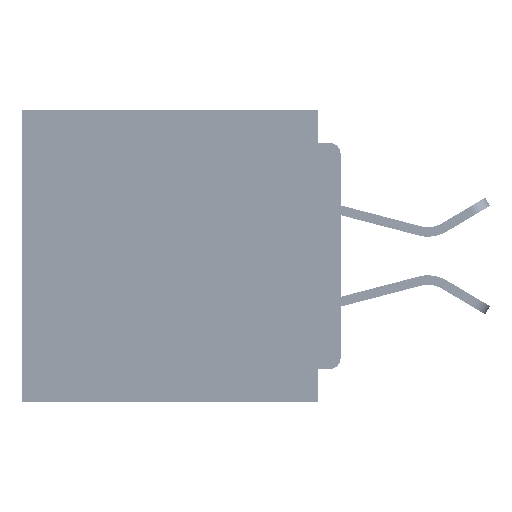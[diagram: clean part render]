
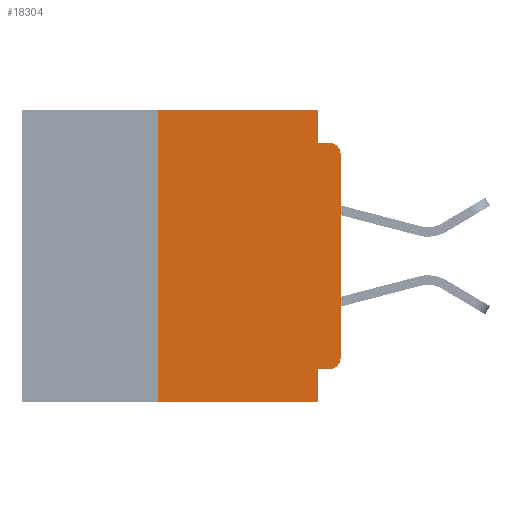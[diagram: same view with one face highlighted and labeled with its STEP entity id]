
A CAD part, left-side view. The second image highlights one B-rep face of the part: STEP entity #18304.
In plain terms, the highlighted planar face has unit normal (-1, 0, 0).
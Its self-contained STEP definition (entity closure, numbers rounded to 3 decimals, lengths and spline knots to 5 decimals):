
#236 = ORIENTED_EDGE ( 'NONE', *, *, #32184, .T. ) ;
#1156 = VERTEX_POINT ( 'NONE', #45394 ) ;
#2224 = ORIENTED_EDGE ( 'NONE', *, *, #14441, .F. ) ;
#2262 = LINE ( 'NONE', #34081, #57100 ) ;
#6101 = VERTEX_POINT ( 'NONE', #47348 ) ;
#6342 = ORIENTED_EDGE ( 'NONE', *, *, #63962, .F. ) ;
#6578 = DIRECTION ( 'NONE',  ( 0., 0., -1. ) ) ;
#8462 = VERTEX_POINT ( 'NONE', #50744 ) ;
#9074 = DIRECTION ( 'NONE',  ( 0., 0., -1. ) ) ;
#9329 = VERTEX_POINT ( 'NONE', #69823 ) ;
#13251 = LINE ( 'NONE', #45003, #56985 ) ;
#14441 = EDGE_CURVE ( 'NONE', #62537, #6101, #2262, .T. ) ;
#14449 = ORIENTED_EDGE ( 'NONE', *, *, #30788, .F. ) ;
#14772 = CARTESIAN_POINT ( 'NONE',  ( 0., 0.031, -0.4 ) ) ;
#15484 = VERTEX_POINT ( 'NONE', #60192 ) ;
#16236 = EDGE_CURVE ( 'NONE', #1156, #57946, #32919, .T. ) ;
#17476 = DIRECTION ( 'NONE',  ( 0., -1., 0. ) ) ;
#17561 = VECTOR ( 'NONE', #68040, 39.37008 ) ;
#18009 = DIRECTION ( 'NONE',  ( -1., 0., 0. ) ) ;
#18274 = VECTOR ( 'NONE', #17476, 39.37008 ) ;
#18304 = ADVANCED_FACE ( 'NONE', ( #35340 ), #30958, .F. ) ;
#18717 = CARTESIAN_POINT ( 'NONE',  ( 0., 0., -0.06 ) ) ;
#18816 = VECTOR ( 'NONE', #20303, 39.37008 ) ;
#18832 = CARTESIAN_POINT ( 'NONE',  ( 0., 0., -0.355 ) ) ;
#20011 = VECTOR ( 'NONE', #60569, 39.37008 ) ;
#20154 = CIRCLE ( 'NONE', #34259, 0.015 ) ;
#20303 = DIRECTION ( 'NONE',  ( 0., 0., -1. ) ) ;
#21872 = LINE ( 'NONE', #59383, #62013 ) ;
#22341 = CARTESIAN_POINT ( 'NONE',  ( 0., 0.25, -0.4 ) ) ;
#22811 = DIRECTION ( 'NONE',  ( 0., 0., 1. ) ) ;
#25427 = CARTESIAN_POINT ( 'NONE',  ( 0., 0.437, 0. ) ) ;
#26601 = CARTESIAN_POINT ( 'NONE',  ( 0., 0.25, 0. ) ) ;
#28005 = AXIS2_PLACEMENT_3D ( 'NONE', #50882, #18009, #56341 ) ;
#28533 = DIRECTION ( 'NONE',  ( 0., -1., 0. ) ) ;
#29160 = ORIENTED_EDGE ( 'NONE', *, *, #61108, .F. ) ;
#29450 = ORIENTED_EDGE ( 'NONE', *, *, #44768, .T. ) ;
#29690 = CARTESIAN_POINT ( 'NONE',  ( 0., 0., -0.34 ) ) ;
#30630 = DIRECTION ( 'NONE',  ( -1., 0., 0. ) ) ;
#30788 = EDGE_CURVE ( 'NONE', #6101, #8462, #13251, .T. ) ;
#30958 = PLANE ( 'NONE',  #44777 ) ;
#32147 = DIRECTION ( 'NONE',  ( 0., -1., 0. ) ) ;
#32184 = EDGE_CURVE ( 'NONE', #70499, #42153, #56794, .T. ) ;
#32205 = LINE ( 'NONE', #18832, #17561 ) ;
#32885 = LINE ( 'NONE', #22341, #20011 ) ;
#32919 = LINE ( 'NONE', #50360, #18274 ) ;
#34081 = CARTESIAN_POINT ( 'NONE',  ( 0., 0.437, 0. ) ) ;
#34259 = AXIS2_PLACEMENT_3D ( 'NONE', #63284, #30630, #68730 ) ;
#35340 = FACE_OUTER_BOUND ( 'NONE', #52729, .T. ) ;
#38305 = CARTESIAN_POINT ( 'NONE',  ( 0., 0.031, -0.4 ) ) ;
#40132 = EDGE_CURVE ( 'NONE', #9329, #70499, #68494, .T. ) ;
#40573 = VECTOR ( 'NONE', #22811, 39.37008 ) ;
#42026 = DIRECTION ( 'NONE',  ( 1., 0., 0. ) ) ;
#42153 = VERTEX_POINT ( 'NONE', #18717 ) ;
#44768 = EDGE_CURVE ( 'NONE', #42153, #63055, #20154, .T. ) ;
#44777 = AXIS2_PLACEMENT_3D ( 'NONE', #25427, #42026, #9074 ) ;
#45003 = CARTESIAN_POINT ( 'NONE',  ( 0., 0.031, 0. ) ) ;
#45394 = CARTESIAN_POINT ( 'NONE',  ( 0., 0.25, -0.4 ) ) ;
#45664 = EDGE_CURVE ( 'NONE', #1156, #62537, #32885, .T. ) ;
#46444 = ORIENTED_EDGE ( 'NONE', *, *, #66779, .F. ) ;
#47348 = CARTESIAN_POINT ( 'NONE',  ( 0., 0.031, 0. ) ) ;
#49178 = ORIENTED_EDGE ( 'NONE', *, *, #16236, .T. ) ;
#50360 = CARTESIAN_POINT ( 'NONE',  ( 0., 0.437, -0.4 ) ) ;
#50744 = CARTESIAN_POINT ( 'NONE',  ( 0., 0.031, -0.045 ) ) ;
#50882 = CARTESIAN_POINT ( 'NONE',  ( 0., 0.015, -0.34 ) ) ;
#52729 = EDGE_LOOP ( 'NONE', ( #236, #29450, #6342, #14449, #2224, #66175, #49178, #46444, #29160, #55626 ) ) ;
#55626 = ORIENTED_EDGE ( 'NONE', *, *, #40132, .T. ) ;
#56341 = DIRECTION ( 'NONE',  ( 0., 0., -1. ) ) ;
#56794 = LINE ( 'NONE', #61023, #40573 ) ;
#56985 = VECTOR ( 'NONE', #6578, 39.37008 ) ;
#57100 = VECTOR ( 'NONE', #28533, 39.37008 ) ;
#57946 = VERTEX_POINT ( 'NONE', #38305 ) ;
#58095 = CARTESIAN_POINT ( 'NONE',  ( 0., 0.015, -0.045 ) ) ;
#59383 = CARTESIAN_POINT ( 'NONE',  ( 0., 0., -0.045 ) ) ;
#60192 = CARTESIAN_POINT ( 'NONE',  ( 0., 0.031, -0.355 ) ) ;
#60569 = DIRECTION ( 'NONE',  ( 0., 0., 1. ) ) ;
#61023 = CARTESIAN_POINT ( 'NONE',  ( 0., 0., 0. ) ) ;
#61108 = EDGE_CURVE ( 'NONE', #9329, #15484, #32205, .T. ) ;
#62013 = VECTOR ( 'NONE', #32147, 39.37008 ) ;
#62427 = LINE ( 'NONE', #14772, #18816 ) ;
#62537 = VERTEX_POINT ( 'NONE', #26601 ) ;
#63055 = VERTEX_POINT ( 'NONE', #58095 ) ;
#63284 = CARTESIAN_POINT ( 'NONE',  ( 0., 0.015, -0.06 ) ) ;
#63962 = EDGE_CURVE ( 'NONE', #8462, #63055, #21872, .T. ) ;
#66175 = ORIENTED_EDGE ( 'NONE', *, *, #45664, .F. ) ;
#66779 = EDGE_CURVE ( 'NONE', #15484, #57946, #62427, .T. ) ;
#68040 = DIRECTION ( 'NONE',  ( 0., 1., 0. ) ) ;
#68494 = CIRCLE ( 'NONE', #28005, 0.015 ) ;
#68730 = DIRECTION ( 'NONE',  ( 0., 0., -1. ) ) ;
#69823 = CARTESIAN_POINT ( 'NONE',  ( 0., 0.015, -0.355 ) ) ;
#70499 = VERTEX_POINT ( 'NONE', #29690 ) ;
